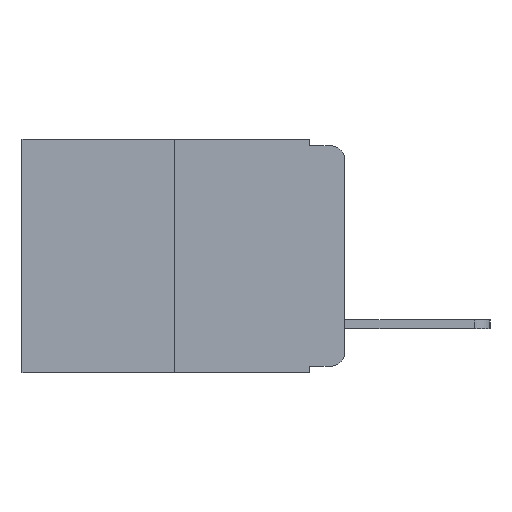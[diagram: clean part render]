
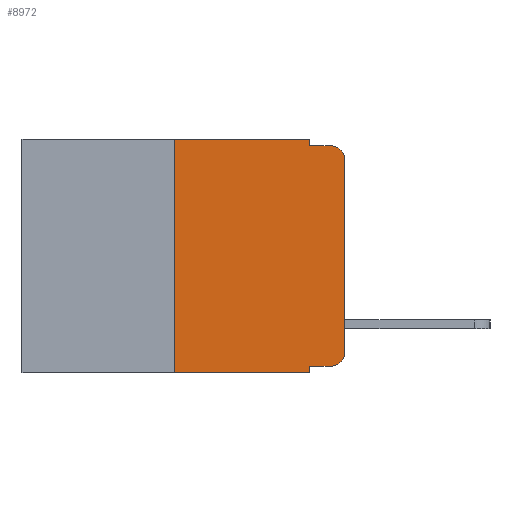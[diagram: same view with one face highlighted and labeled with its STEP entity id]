
A CAD part, left-side view. The second image highlights one B-rep face of the part: STEP entity #8972.
In plain terms, the highlighted planar face has unit normal (-1, 0, 0).
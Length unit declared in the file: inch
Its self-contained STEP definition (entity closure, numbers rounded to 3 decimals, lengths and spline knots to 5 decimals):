
#463 = VERTEX_POINT ( 'NONE', #15336 ) ;
#1028 = ORIENTED_EDGE ( 'NONE', *, *, #4108, .T. ) ;
#1218 = DIRECTION ( 'NONE',  ( 0., 0., -1. ) ) ;
#1501 = VERTEX_POINT ( 'NONE', #3403 ) ;
#1588 = ORIENTED_EDGE ( 'NONE', *, *, #8439, .F. ) ;
#1779 = PLANE ( 'NONE',  #15195 ) ;
#1793 = CARTESIAN_POINT ( 'NONE',  ( 0., 0.051, 0. ) ) ;
#1827 = VERTEX_POINT ( 'NONE', #4355 ) ;
#2247 = CARTESIAN_POINT ( 'NONE',  ( 0., 0.051, -0.333 ) ) ;
#2265 = DIRECTION ( 'NONE',  ( 0., 0., 1. ) ) ;
#2485 = VECTOR ( 'NONE', #7683, 39.37008 ) ;
#2682 = VECTOR ( 'NONE', #2265, 39.37008 ) ;
#2787 = VECTOR ( 'NONE', #15538, 39.37008 ) ;
#2937 = ORIENTED_EDGE ( 'NONE', *, *, #9028, .F. ) ;
#3403 = CARTESIAN_POINT ( 'NONE',  ( 0., 0.051, 0. ) ) ;
#3515 = CARTESIAN_POINT ( 'NONE',  ( 0., 0.473, 0. ) ) ;
#3831 = EDGE_CURVE ( 'NONE', #11077, #463, #8104, .T. ) ;
#4108 = EDGE_CURVE ( 'NONE', #8546, #6372, #15060, .T. ) ;
#4179 = VERTEX_POINT ( 'NONE', #10357 ) ;
#4220 = CARTESIAN_POINT ( 'NONE',  ( 0., 0.051, -0.01 ) ) ;
#4355 = CARTESIAN_POINT ( 'NONE',  ( 0., 0.25, 0. ) ) ;
#4762 = ORIENTED_EDGE ( 'NONE', *, *, #15043, .T. ) ;
#4954 = EDGE_CURVE ( 'NONE', #16830, #11077, #7231, .T. ) ;
#5025 = DIRECTION ( 'NONE',  ( 0., -1., 0. ) ) ;
#5205 = DIRECTION ( 'NONE',  ( 0., 0., -1. ) ) ;
#5300 = ORIENTED_EDGE ( 'NONE', *, *, #13971, .T. ) ;
#5584 = DIRECTION ( 'NONE',  ( 0., -1., 0. ) ) ;
#5760 = VECTOR ( 'NONE', #15936, 39.37008 ) ;
#6116 = ORIENTED_EDGE ( 'NONE', *, *, #4954, .T. ) ;
#6372 = VERTEX_POINT ( 'NONE', #10400 ) ;
#6656 = ORIENTED_EDGE ( 'NONE', *, *, #3831, .T. ) ;
#6735 = VECTOR ( 'NONE', #5025, 39.37008 ) ;
#7093 = CARTESIAN_POINT ( 'NONE',  ( 0., 0.473, 0. ) ) ;
#7231 = LINE ( 'NONE', #2247, #7775 ) ;
#7453 = EDGE_LOOP ( 'NONE', ( #4762, #5300, #10410, #14726, #2937, #13982, #1028, #1588, #6116, #6656 ) ) ;
#7683 = DIRECTION ( 'NONE',  ( 0., 0., 1. ) ) ;
#7743 = LINE ( 'NONE', #15680, #2682 ) ;
#7775 = VECTOR ( 'NONE', #5584, 39.37008 ) ;
#8030 = CARTESIAN_POINT ( 'NONE',  ( 0., 0.051, 0. ) ) ;
#8104 = CIRCLE ( 'NONE', #14463, 0.02 ) ;
#8190 = DIRECTION ( 'NONE',  ( -1., 0., 0. ) ) ;
#8439 = EDGE_CURVE ( 'NONE', #16830, #6372, #11824, .T. ) ;
#8546 = VERTEX_POINT ( 'NONE', #14168 ) ;
#8972 = ADVANCED_FACE ( 'NONE', ( #14059 ), #1779, .F. ) ;
#9028 = EDGE_CURVE ( 'NONE', #1827, #1501, #17400, .T. ) ;
#9170 = VECTOR ( 'NONE', #18604, 39.37008 ) ;
#9191 = CARTESIAN_POINT ( 'NONE',  ( 0., 0.02, -0.333 ) ) ;
#9399 = DIRECTION ( 'NONE',  ( -1., 0., 0. ) ) ;
#9794 = LINE ( 'NONE', #4220, #5760 ) ;
#10357 = CARTESIAN_POINT ( 'NONE',  ( 0., 0.051, -0.01 ) ) ;
#10400 = CARTESIAN_POINT ( 'NONE',  ( 0., 0.051, -0.343 ) ) ;
#10410 = ORIENTED_EDGE ( 'NONE', *, *, #12893, .F. ) ;
#10651 = VECTOR ( 'NONE', #1218, 39.37008 ) ;
#10717 = EDGE_CURVE ( 'NONE', #8546, #1827, #7743, .T. ) ;
#11077 = VERTEX_POINT ( 'NONE', #9191 ) ;
#11543 = LINE ( 'NONE', #14215, #2485 ) ;
#11815 = EDGE_CURVE ( 'NONE', #1501, #4179, #14954, .T. ) ;
#11824 = LINE ( 'NONE', #1793, #2787 ) ;
#12893 = EDGE_CURVE ( 'NONE', #4179, #20046, #9794, .T. ) ;
#13868 = VERTEX_POINT ( 'NONE', #16134 ) ;
#13971 = EDGE_CURVE ( 'NONE', #13868, #20046, #18719, .T. ) ;
#13982 = ORIENTED_EDGE ( 'NONE', *, *, #10717, .F. ) ;
#14059 = FACE_OUTER_BOUND ( 'NONE', #7453, .T. ) ;
#14168 = CARTESIAN_POINT ( 'NONE',  ( 0., 0.25, -0.343 ) ) ;
#14215 = CARTESIAN_POINT ( 'NONE',  ( 0., 0., 0. ) ) ;
#14463 = AXIS2_PLACEMENT_3D ( 'NONE', #19224, #9399, #20823 ) ;
#14726 = ORIENTED_EDGE ( 'NONE', *, *, #11815, .F. ) ;
#14954 = LINE ( 'NONE', #8030, #10651 ) ;
#15043 = EDGE_CURVE ( 'NONE', #463, #13868, #11543, .T. ) ;
#15060 = LINE ( 'NONE', #16709, #6735 ) ;
#15141 = AXIS2_PLACEMENT_3D ( 'NONE', #18061, #8190, #19693 ) ;
#15195 = AXIS2_PLACEMENT_3D ( 'NONE', #3515, #15218, #5205 ) ;
#15218 = DIRECTION ( 'NONE',  ( 1., 0., 0. ) ) ;
#15336 = CARTESIAN_POINT ( 'NONE',  ( 0., 0., -0.313 ) ) ;
#15538 = DIRECTION ( 'NONE',  ( 0., 0., -1. ) ) ;
#15680 = CARTESIAN_POINT ( 'NONE',  ( 0., 0.25, 0. ) ) ;
#15936 = DIRECTION ( 'NONE',  ( 0., -1., 0. ) ) ;
#16134 = CARTESIAN_POINT ( 'NONE',  ( 0., 0., -0.03 ) ) ;
#16709 = CARTESIAN_POINT ( 'NONE',  ( 0., 0.473, -0.343 ) ) ;
#16830 = VERTEX_POINT ( 'NONE', #16968 ) ;
#16968 = CARTESIAN_POINT ( 'NONE',  ( 0., 0.051, -0.333 ) ) ;
#17400 = LINE ( 'NONE', #7093, #9170 ) ;
#18061 = CARTESIAN_POINT ( 'NONE',  ( 0., 0.02, -0.03 ) ) ;
#18604 = DIRECTION ( 'NONE',  ( 0., -1., 0. ) ) ;
#18719 = CIRCLE ( 'NONE', #15141, 0.02 ) ;
#19224 = CARTESIAN_POINT ( 'NONE',  ( 0., 0.02, -0.313 ) ) ;
#19273 = CARTESIAN_POINT ( 'NONE',  ( 0., 0.02, -0.01 ) ) ;
#19693 = DIRECTION ( 'NONE',  ( 0., 0., -1. ) ) ;
#20046 = VERTEX_POINT ( 'NONE', #19273 ) ;
#20823 = DIRECTION ( 'NONE',  ( 0., 0., -1. ) ) ;
